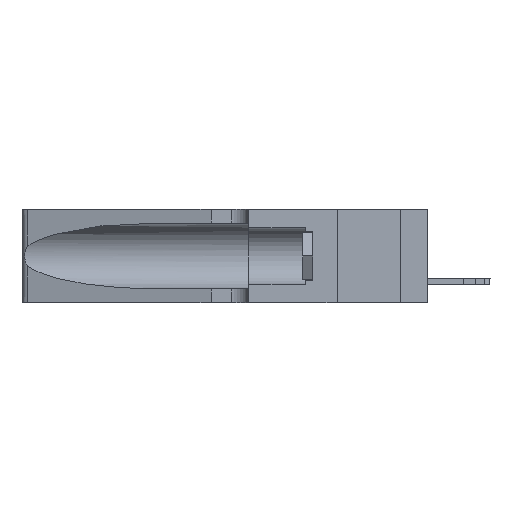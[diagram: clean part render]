
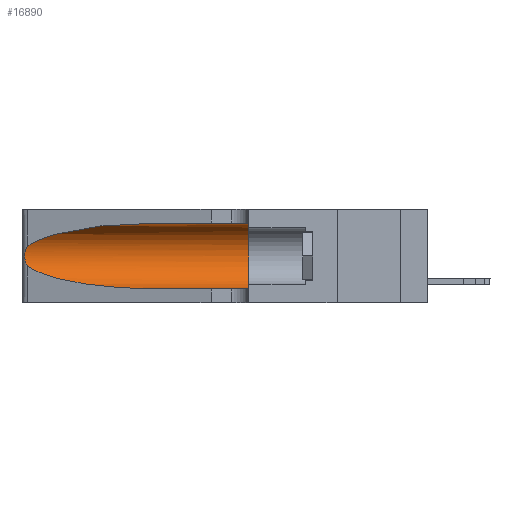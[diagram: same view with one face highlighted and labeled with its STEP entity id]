
A CAD part, left-side view. The second image highlights one B-rep face of the part: STEP entity #16890.
In plain terms, the highlighted cylindrical face has radius 3.308 mm (diameter 6.617 mm), a partial arc.
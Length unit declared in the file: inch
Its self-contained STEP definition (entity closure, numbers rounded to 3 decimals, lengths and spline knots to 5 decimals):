
#133 = VERTEX_POINT ( 'NONE', #13816 ) ;
#289 = CARTESIAN_POINT ( 'NONE',  ( 0.25854, 1.2359, 0.20912 ) ) ;
#316 = EDGE_CURVE ( 'NONE', #783, #133, #533, .T. ) ;
#533 = CIRCLE ( 'NONE', #6480, 0.13025 ) ;
#598 = EDGE_CURVE ( 'NONE', #1892, #133, #2519, .T. ) ;
#673 = DIRECTION ( 'NONE',  ( 0., 0., -1. ) ) ;
#783 = VERTEX_POINT ( 'NONE', #3566 ) ;
#1213 = FACE_OUTER_BOUND ( 'NONE', #11911, .T. ) ;
#1550 = CARTESIAN_POINT ( 'NONE',  ( 0.26017, 1.23833, 0.17102 ) ) ;
#1862 = AXIS2_PLACEMENT_3D ( 'NONE', #14727, #5016, #673 ) ;
#1892 = VERTEX_POINT ( 'NONE', #14640 ) ;
#2042 = DIRECTION ( 'NONE',  ( 0., -1., 0. ) ) ;
#2519 = LINE ( 'NONE', #8851, #5852 ) ;
#3029 =( BOUNDED_CURVE ( )  B_SPLINE_CURVE ( 3, ( #12257, #10941, #6701, #8137 ),
 .UNSPECIFIED., .F., .T. ) 
 B_SPLINE_CURVE_WITH_KNOTS ( ( 4, 4 ),
 ( 1.5708, 2.84003 ),
 .UNSPECIFIED. ) 
 CURVE ( )  GEOMETRIC_REPRESENTATION_ITEM ( )  RATIONAL_B_SPLINE_CURVE ( ( 1., 0.87, 0.87, 1. ) ) 
 REPRESENTATION_ITEM ( '' )  );
#3539 = EDGE_CURVE ( 'NONE', #9483, #14791, #3029, .T. ) ;
#3566 = CARTESIAN_POINT ( 'NONE',  ( 0.1305, 0.35, 0.31525 ) ) ;
#4282 = CARTESIAN_POINT ( 'NONE',  ( 0.1305, 0.35, 0.185 ) ) ;
#4386 = CARTESIAN_POINT ( 'NONE',  ( 0.25487, 1.22718, 0.22369 ) ) ;
#4510 = CARTESIAN_POINT ( 'NONE',  ( 0.26018, 1.23835, 0.19895 ) ) ;
#5016 = DIRECTION ( 'NONE',  ( 0., -1., 0. ) ) ;
#5254 = LINE ( 'NONE', #13488, #12130 ) ;
#5451 = CARTESIAN_POINT ( 'NONE',  ( 0.2373, 1.15595, 0.08982 ) ) ;
#5696 = CARTESIAN_POINT ( 'NONE',  ( 0.26075, 1.23896, 0.178 ) ) ;
#5816 = CARTESIAN_POINT ( 'NONE',  ( 0.25487, 1.22718, 0.14631 ) ) ;
#5852 = VECTOR ( 'NONE', #2042, 39.37008 ) ;
#5941 = CARTESIAN_POINT ( 'NONE',  ( 0.25639, 1.23186, 0.15144 ) ) ;
#6204 = ORIENTED_EDGE ( 'NONE', *, *, #14940, .T. ) ;
#6333 = CARTESIAN_POINT ( 'NONE',  ( 0.25487, 1.22718, 0.22369 ) ) ;
#6480 = AXIS2_PLACEMENT_3D ( 'NONE', #4282, #8334, #7033 ) ;
#6701 = CARTESIAN_POINT ( 'NONE',  ( 0.2373, 1.15595, 0.28018 ) ) ;
#6820 = CARTESIAN_POINT ( 'NONE',  ( 0.25487, 1.22718, 0.14631 ) ) ;
#6920 = B_SPLINE_CURVE_WITH_KNOTS ( 'NONE', 3,
 ( #4386, #14288, #7208, #12988, #289, #4510, #10005, #5696, #1550, #15718, #8718, #5941, #12747, #5816 ),
 .UNSPECIFIED., .F., .F.,
 ( 4, 2, 2, 2, 2, 2, 4 ),
 ( 0., 0.00027, 0.00053, 0.00107, 0.0016, 0.00187, 0.00214 ),
 .UNSPECIFIED. ) ;
#7033 = DIRECTION ( 'NONE',  ( 0., 0., 1. ) ) ;
#7208 = CARTESIAN_POINT ( 'NONE',  ( 0.25639, 1.23184, 0.21858 ) ) ;
#8137 = CARTESIAN_POINT ( 'NONE',  ( 0.25487, 1.22718, 0.22369 ) ) ;
#8138 = ORIENTED_EDGE ( 'NONE', *, *, #3539, .T. ) ;
#8334 = DIRECTION ( 'NONE',  ( 0., 1., 0. ) ) ;
#8347 = ORIENTED_EDGE ( 'NONE', *, *, #316, .F. ) ;
#8376 = CARTESIAN_POINT ( 'NONE',  ( 0.1305, 0.72297, 0.05475 ) ) ;
#8718 = CARTESIAN_POINT ( 'NONE',  ( 0.25789, 1.23486, 0.15765 ) ) ;
#8851 = CARTESIAN_POINT ( 'NONE',  ( 0.1305, 1.61858, 0.05475 ) ) ;
#9483 = VERTEX_POINT ( 'NONE', #17561 ) ;
#10005 = CARTESIAN_POINT ( 'NONE',  ( 0.26075, 1.23896, 0.19203 ) ) ;
#10211 = EDGE_CURVE ( 'NONE', #14791, #11686, #6920, .T. ) ;
#10941 = CARTESIAN_POINT ( 'NONE',  ( 0.18966, 0.96281, 0.31525 ) ) ;
#11500 = ORIENTED_EDGE ( 'NONE', *, *, #10211, .T. ) ;
#11686 = VERTEX_POINT ( 'NONE', #12041 ) ;
#11911 = EDGE_LOOP ( 'NONE', ( #8138, #11500, #6204, #16902, #8347, #14970 ) ) ;
#12041 = CARTESIAN_POINT ( 'NONE',  ( 0.25487, 1.22718, 0.14631 ) ) ;
#12130 = VECTOR ( 'NONE', #17790, 39.37008 ) ;
#12257 = CARTESIAN_POINT ( 'NONE',  ( 0.1305, 0.72297, 0.31525 ) ) ;
#12747 = CARTESIAN_POINT ( 'NONE',  ( 0.25555, 1.22993, 0.14849 ) ) ;
#12988 = CARTESIAN_POINT ( 'NONE',  ( 0.25787, 1.23484, 0.2124 ) ) ;
#13488 = CARTESIAN_POINT ( 'NONE',  ( 0.1305, 1.61858, 0.31525 ) ) ;
#13804 = EDGE_CURVE ( 'NONE', #9483, #783, #5254, .T. ) ;
#13816 = CARTESIAN_POINT ( 'NONE',  ( 0.1305, 0.35, 0.05475 ) ) ;
#14288 = CARTESIAN_POINT ( 'NONE',  ( 0.25555, 1.22994, 0.2215 ) ) ;
#14640 = CARTESIAN_POINT ( 'NONE',  ( 0.1305, 0.72297, 0.05475 ) ) ;
#14727 = CARTESIAN_POINT ( 'NONE',  ( 0.1305, 1.61858, 0.185 ) ) ;
#14791 = VERTEX_POINT ( 'NONE', #6333 ) ;
#14940 = EDGE_CURVE ( 'NONE', #11686, #1892, #16208, .T. ) ;
#14970 = ORIENTED_EDGE ( 'NONE', *, *, #13804, .F. ) ;
#15718 = CARTESIAN_POINT ( 'NONE',  ( 0.25856, 1.23593, 0.16098 ) ) ;
#15818 = CYLINDRICAL_SURFACE ( 'NONE', #1862, 0.13025 ) ;
#16208 =( BOUNDED_CURVE ( )  B_SPLINE_CURVE ( 3, ( #6820, #5451, #16670, #8376 ),
 .UNSPECIFIED., .F., .T. ) 
 B_SPLINE_CURVE_WITH_KNOTS ( ( 4, 4 ),
 ( 3.44316, 4.71239 ),
 .UNSPECIFIED. ) 
 CURVE ( )  GEOMETRIC_REPRESENTATION_ITEM ( )  RATIONAL_B_SPLINE_CURVE ( ( 1., 0.87, 0.87, 1. ) ) 
 REPRESENTATION_ITEM ( '' )  );
#16670 = CARTESIAN_POINT ( 'NONE',  ( 0.18966, 0.96281, 0.05475 ) ) ;
#16890 = ADVANCED_FACE ( 'NONE', ( #1213 ), #15818, .F. ) ;
#16902 = ORIENTED_EDGE ( 'NONE', *, *, #598, .T. ) ;
#17561 = CARTESIAN_POINT ( 'NONE',  ( 0.1305, 0.72297, 0.31525 ) ) ;
#17790 = DIRECTION ( 'NONE',  ( 0., -1., 0. ) ) ;
